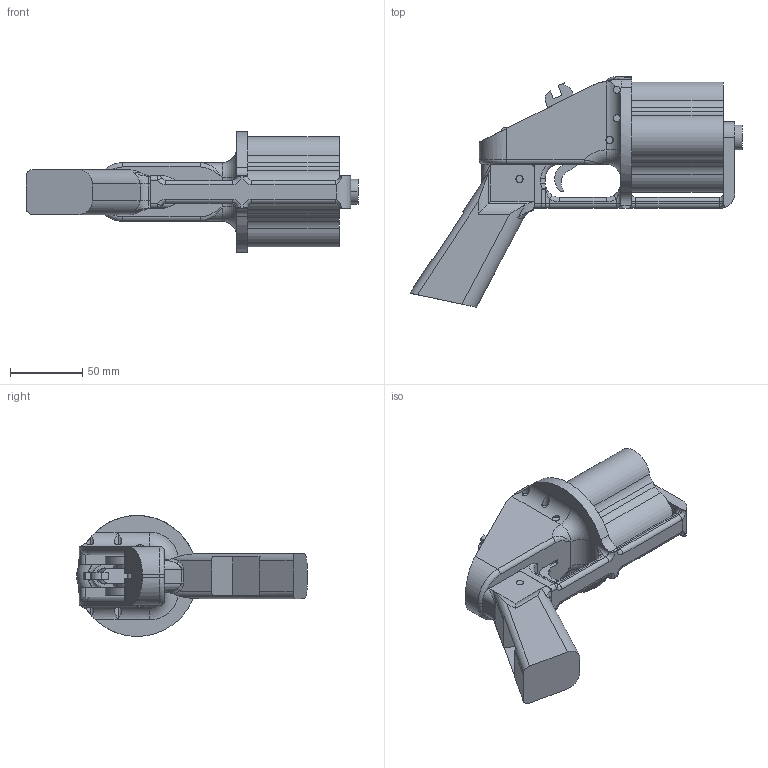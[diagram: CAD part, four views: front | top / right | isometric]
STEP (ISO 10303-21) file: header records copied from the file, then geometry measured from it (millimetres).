
FILE_DESCRIPTION (( 'STEP AP214' ), '1' );
FILE_NAME ('LiberatorSWNative.STEP', '2013-06-07T17:14:15', ( 'Asher' ), ( '' ), 'SwSTEP 2.0', 'SolidWorks 2013', '' );
FILE_SCHEMA (( 'AUTOMOTIVE_DESIGN' ));
Length unit declared in the file: inch
Products named in the file (17): LiberatorSWNative; MainRod^LiberatorSWNative; hammer_pin; trigger_spring; HammerSpringAssem; spring_connecting_rod; spring_connecting_rod_bushing; Spring; 4shot_380_barrel_revolver; frame_pins_(x3); grip_pin; firing_pin_bushing; GripRemodeled; trigger; hammer; hammer_body; frame_(no_sn)
Assembly tree (19 placements, depth 3):
  LiberatorSWNative
    frame_(no_sn)
    hammer_body
    hammer
    trigger
    GripRemodeled
    firing_pin_bushing
    grip_pin
    frame_pins_(x3)  x3
    4shot_380_barrel_revolver
    HammerSpringAssem
      Spring  x2
      spring_connecting_rod_bushing
      spring_connecting_rod
    trigger_spring
    hammer_pin
    MainRod^LiberatorSWNative
Bounding box: 229.99 x 159.69 x 83.81 mm (x, y, z)
Volume: 476265.5 mm3; surface area: 126344.4 mm2
Topology: 18 solids, 18 shells, 668 faces, 1775 edges, 1142 vertices
Faces by surface type: plane 306, cylinder 276, torus 58, bspline 24, sphere 4
Entity records: 23226 total; most frequent: CARTESIAN_POINT 6128, DIRECTION 3453, ORIENTED_EDGE 3442, EDGE_CURVE 1721, AXIS2_PLACEMENT_3D 1270, VERTEX_POINT 1110, LINE 913, VECTOR 913
